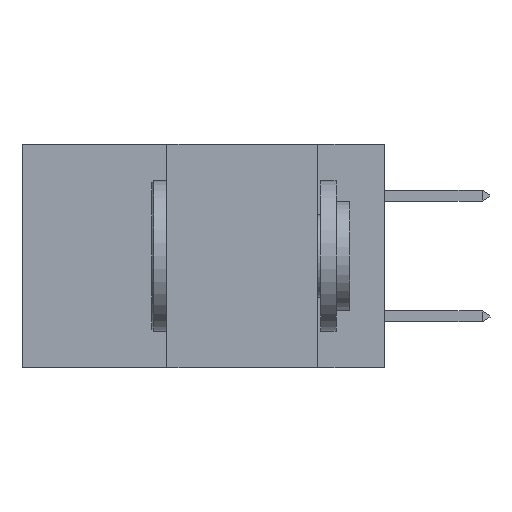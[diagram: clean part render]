
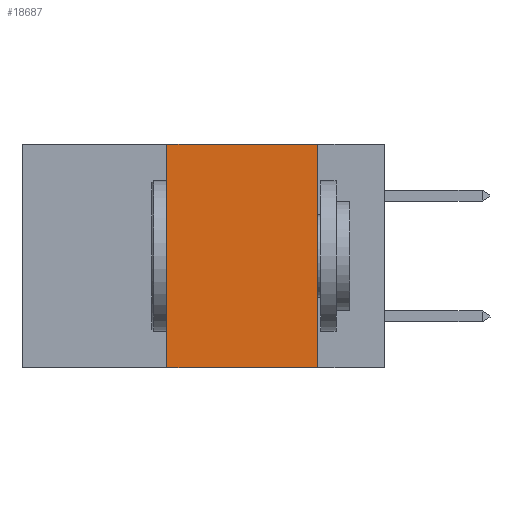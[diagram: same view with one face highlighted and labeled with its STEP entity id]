
A CAD part, left-side view. The second image highlights one B-rep face of the part: STEP entity #18687.
In plain terms, the highlighted planar face has unit normal (-1, 0, 0).
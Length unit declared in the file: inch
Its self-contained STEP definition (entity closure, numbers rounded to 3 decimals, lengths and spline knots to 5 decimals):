
#1836 = DIRECTION ( 'NONE',  ( 0., 0., -1. ) ) ;
#2306 = LINE ( 'NONE', #7028, #16115 ) ;
#2837 = ORIENTED_EDGE ( 'NONE', *, *, #4293, .T. ) ;
#3033 = AXIS2_PLACEMENT_3D ( 'NONE', #23357, #12708, #1836 ) ;
#4293 = EDGE_CURVE ( 'NONE', #13249, #16460, #6238, .T. ) ;
#4309 = CARTESIAN_POINT ( 'NONE',  ( 0., 0.11, 0. ) ) ;
#4608 = CARTESIAN_POINT ( 'NONE',  ( 0., 0.11, -0.37 ) ) ;
#4773 = VECTOR ( 'NONE', #11018, 39.37008 ) ;
#5179 = DIRECTION ( 'NONE',  ( 0., 0., -1. ) ) ;
#5446 = ORIENTED_EDGE ( 'NONE', *, *, #15494, .F. ) ;
#5524 = PLANE ( 'NONE',  #3033 ) ;
#5829 = FACE_OUTER_BOUND ( 'NONE', #7467, .T. ) ;
#6238 = LINE ( 'NONE', #9470, #19260 ) ;
#7028 = CARTESIAN_POINT ( 'NONE',  ( 0., 0.11, 0. ) ) ;
#7320 = LINE ( 'NONE', #17300, #16139 ) ;
#7467 = EDGE_LOOP ( 'NONE', ( #5446, #16700, #19284, #2837 ) ) ;
#9304 = DIRECTION ( 'NONE',  ( 0., -1., 0. ) ) ;
#9470 = CARTESIAN_POINT ( 'NONE',  ( 0., 0.6, -0.37 ) ) ;
#9632 = LINE ( 'NONE', #12766, #4773 ) ;
#9804 = VERTEX_POINT ( 'NONE', #4309 ) ;
#11018 = DIRECTION ( 'NONE',  ( 0., 0., 1. ) ) ;
#12706 = VERTEX_POINT ( 'NONE', #20490 ) ;
#12708 = DIRECTION ( 'NONE',  ( 1., 0., 0. ) ) ;
#12766 = CARTESIAN_POINT ( 'NONE',  ( 0., 0.36, 0. ) ) ;
#13249 = VERTEX_POINT ( 'NONE', #18509 ) ;
#15494 = EDGE_CURVE ( 'NONE', #9804, #16460, #2306, .T. ) ;
#16115 = VECTOR ( 'NONE', #5179, 39.37008 ) ;
#16139 = VECTOR ( 'NONE', #19064, 39.37008 ) ;
#16460 = VERTEX_POINT ( 'NONE', #4608 ) ;
#16700 = ORIENTED_EDGE ( 'NONE', *, *, #18427, .F. ) ;
#17300 = CARTESIAN_POINT ( 'NONE',  ( 0., 0.6, 0. ) ) ;
#17441 = EDGE_CURVE ( 'NONE', #13249, #12706, #9632, .T. ) ;
#18427 = EDGE_CURVE ( 'NONE', #12706, #9804, #7320, .T. ) ;
#18509 = CARTESIAN_POINT ( 'NONE',  ( 0., 0.36, -0.37 ) ) ;
#18687 = ADVANCED_FACE ( 'NONE', ( #5829 ), #5524, .F. ) ;
#19064 = DIRECTION ( 'NONE',  ( 0., -1., 0. ) ) ;
#19260 = VECTOR ( 'NONE', #9304, 39.37008 ) ;
#19284 = ORIENTED_EDGE ( 'NONE', *, *, #17441, .F. ) ;
#20490 = CARTESIAN_POINT ( 'NONE',  ( 0., 0.36, 0. ) ) ;
#23357 = CARTESIAN_POINT ( 'NONE',  ( 0., 0.6, 0. ) ) ;
